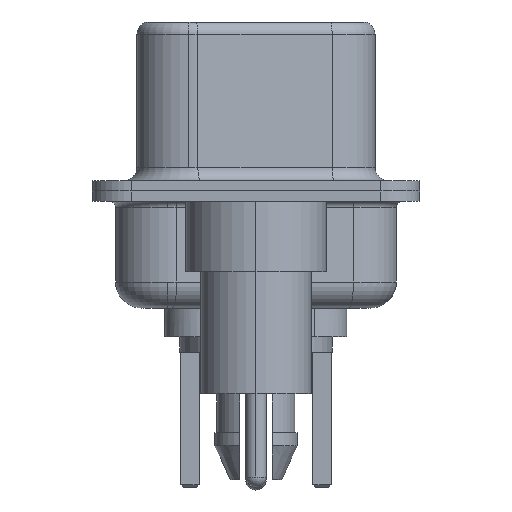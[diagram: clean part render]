
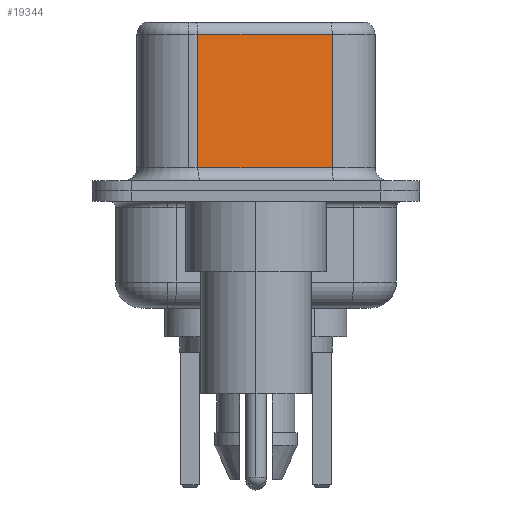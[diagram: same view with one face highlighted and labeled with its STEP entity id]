
A CAD part, left-side view. The second image highlights one B-rep face of the part: STEP entity #19344.
In plain terms, the highlighted planar face has unit normal (-0.985, -0.174, 0).
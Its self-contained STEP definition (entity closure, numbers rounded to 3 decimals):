
#49 = VECTOR ( 'NONE', #20165, 1000. ) ;
#1466 = EDGE_CURVE ( 'NONE', #9818, #21524, #9494, .T. ) ;
#1561 = ORIENTED_EDGE ( 'NONE', *, *, #23610, .T. ) ;
#2871 = VECTOR ( 'NONE', #13403, 1000. ) ;
#3222 = CARTESIAN_POINT ( 'NONE',  ( 3.655, 2.233, 6.02 ) ) ;
#3227 = CARTESIAN_POINT ( 'NONE',  ( 4.565, -2.927, 6.02 ) ) ;
#3838 = AXIS2_PLACEMENT_3D ( 'NONE', #12024, #23558, #12094 ) ;
#4430 = VERTEX_POINT ( 'NONE', #3227 ) ;
#7497 = ORIENTED_EDGE ( 'NONE', *, *, #11793, .F. ) ;
#8677 = CARTESIAN_POINT ( 'NONE',  ( 3.655, 2.233, 0.9 ) ) ;
#9063 = CARTESIAN_POINT ( 'NONE',  ( 4.565, -2.927, 0.9 ) ) ;
#9494 = LINE ( 'NONE', #20420, #49 ) ;
#9818 = VERTEX_POINT ( 'NONE', #8677 ) ;
#10454 = VERTEX_POINT ( 'NONE', #3222 ) ;
#10502 = ORIENTED_EDGE ( 'NONE', *, *, #1466, .T. ) ;
#10992 = VECTOR ( 'NONE', #14509, 1000. ) ;
#11793 = EDGE_CURVE ( 'NONE', #4430, #21524, #21147, .T. ) ;
#12024 = CARTESIAN_POINT ( 'NONE',  ( 4.565, -2.927, 6.52 ) ) ;
#12045 = CARTESIAN_POINT ( 'NONE',  ( 4.565, -2.927, 6.02 ) ) ;
#12094 = DIRECTION ( 'NONE',  ( -0.174, 0.985, 0. ) ) ;
#13403 = DIRECTION ( 'NONE',  ( 0., 0., -1. ) ) ;
#14509 = DIRECTION ( 'NONE',  ( 0., 0., -1. ) ) ;
#15797 = DIRECTION ( 'NONE',  ( -0.174, 0.985, 0. ) ) ;
#18080 = LINE ( 'NONE', #19201, #2871 ) ;
#18098 = LINE ( 'NONE', #12045, #22597 ) ;
#18278 = FACE_OUTER_BOUND ( 'NONE', #20726, .T. ) ;
#19130 = ORIENTED_EDGE ( 'NONE', *, *, #24144, .T. ) ;
#19201 = CARTESIAN_POINT ( 'NONE',  ( 3.655, 2.233, 6.52 ) ) ;
#19344 = ADVANCED_FACE ( 'NONE', ( #18278 ), #21637, .F. ) ;
#20165 = DIRECTION ( 'NONE',  ( 0.174, -0.985, 0. ) ) ;
#20420 = CARTESIAN_POINT ( 'NONE',  ( 4.565, -2.927, 0.9 ) ) ;
#20726 = EDGE_LOOP ( 'NONE', ( #7497, #1561, #19130, #10502 ) ) ;
#21147 = LINE ( 'NONE', #22062, #10992 ) ;
#21524 = VERTEX_POINT ( 'NONE', #9063 ) ;
#21637 = PLANE ( 'NONE',  #3838 ) ;
#22062 = CARTESIAN_POINT ( 'NONE',  ( 4.565, -2.927, 6.52 ) ) ;
#22597 = VECTOR ( 'NONE', #15797, 1000. ) ;
#23558 = DIRECTION ( 'NONE',  ( 0.985, 0.174, 0. ) ) ;
#23610 = EDGE_CURVE ( 'NONE', #4430, #10454, #18098, .T. ) ;
#24144 = EDGE_CURVE ( 'NONE', #10454, #9818, #18080, .T. ) ;
